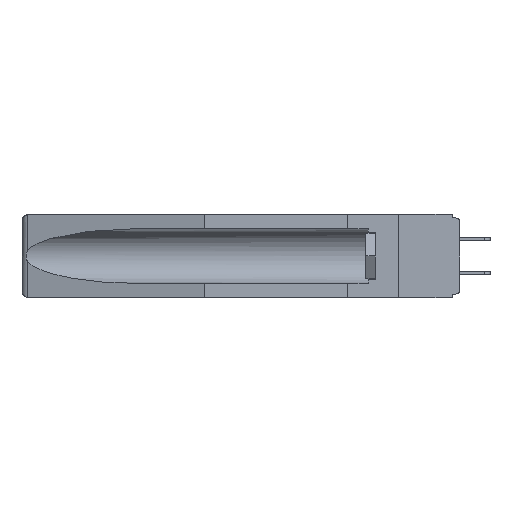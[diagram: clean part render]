
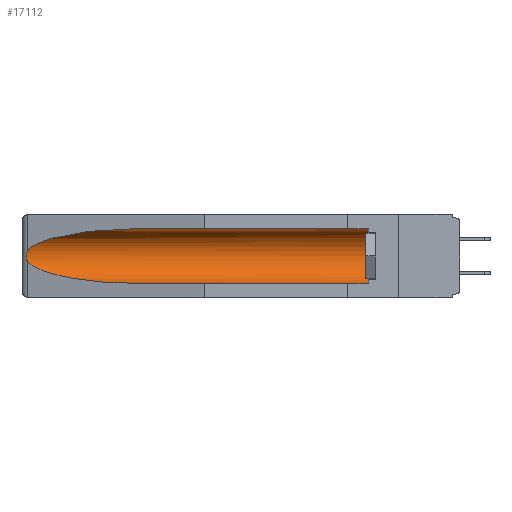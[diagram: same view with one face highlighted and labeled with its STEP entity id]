
A CAD part, left-side view. The second image highlights one B-rep face of the part: STEP entity #17112.
In plain terms, the highlighted cylindrical face has radius 2.857 mm (diameter 5.715 mm), a partial arc.
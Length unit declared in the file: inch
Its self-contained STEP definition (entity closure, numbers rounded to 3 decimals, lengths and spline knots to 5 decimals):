
#149 = VECTOR ( 'NONE', #13962, 39.37008 ) ;
#211 = CARTESIAN_POINT ( 'NONE',  ( 0.26537, 1.52718, -0.19328 ) ) ;
#336 = LINE ( 'NONE', #952, #14127 ) ;
#565 = EDGE_CURVE ( 'NONE', #11553, #15283, #336, .T. ) ;
#869 = CARTESIAN_POINT ( 'NONE',  ( 0.155, 1.07973, -0.284 ) ) ;
#952 = CARTESIAN_POINT ( 'NONE',  ( 0.155, -0.30754, -0.059 ) ) ;
#1368 = ORIENTED_EDGE ( 'NONE', *, *, #20794, .T. ) ;
#1974 = CARTESIAN_POINT ( 'NONE',  ( 0.26597, 1.5296, -0.19026 ) ) ;
#2362 = VERTEX_POINT ( 'NONE', #9225 ) ;
#2895 = AXIS2_PLACEMENT_3D ( 'NONE', #11987, #12065, #15499 ) ;
#2953 = DIRECTION ( 'NONE',  ( 0., 1., 0. ) ) ;
#3411 = ORIENTED_EDGE ( 'NONE', *, *, #19638, .T. ) ;
#3944 = DIRECTION ( 'NONE',  ( 0., 1., 0. ) ) ;
#4261 = ORIENTED_EDGE ( 'NONE', *, *, #10939, .F. ) ;
#4383 = CARTESIAN_POINT ( 'NONE',  ( 0.155, 1.07973, -0.059 ) ) ;
#4725 = CARTESIAN_POINT ( 'NONE',  ( 0.155, 0.126, -0.059 ) ) ;
#4789 = CARTESIAN_POINT ( 'NONE',  ( 0.25451, 1.48313, -0.24835 ) ) ;
#4915 = CARTESIAN_POINT ( 'NONE',  ( 0.26537, 1.52718, -0.14972 ) ) ;
#4972 = EDGE_CURVE ( 'NONE', #11870, #2362, #10192, .T. ) ;
#5327 = CARTESIAN_POINT ( 'NONE',  ( 0.2673, 1.5327, -0.16383 ) ) ;
#5405 = CARTESIAN_POINT ( 'NONE',  ( 0.2673, 1.53269, -0.17917 ) ) ;
#5622 = CARTESIAN_POINT ( 'NONE',  ( 0.26654, 1.53092, -0.15636 ) ) ;
#5827 = CARTESIAN_POINT ( 'NONE',  ( 0.155, -0.30754, -0.1715 ) ) ;
#6804 = CARTESIAN_POINT ( 'NONE',  ( 0.155, 1.07973, -0.284 ) ) ;
#7190 = CARTESIAN_POINT ( 'NONE',  ( 0.26537, 1.52718, -0.14972 ) ) ;
#7293 = ORIENTED_EDGE ( 'NONE', *, *, #565, .T. ) ;
#8412 = AXIS2_PLACEMENT_3D ( 'NONE', #5827, #3944, #18020 ) ;
#8425 = ORIENTED_EDGE ( 'NONE', *, *, #21726, .T. ) ;
#9023 = CARTESIAN_POINT ( 'NONE',  ( 0.2675, 1.53308, -0.17534 ) ) ;
#9225 = CARTESIAN_POINT ( 'NONE',  ( 0.26537, 1.52718, -0.19328 ) ) ;
#10192 = B_SPLINE_CURVE_WITH_KNOTS ( 'NONE', 3,
 ( #7190, #19563, #5622, #5327, #17592, #9023, #5405, #10769, #1974, #211 ),
 .UNSPECIFIED., .F., .F.,
 ( 4, 2, 2, 2, 4 ),
 ( 0., 0.00029, 0.00058, 0.00087, 0.00117 ),
 .UNSPECIFIED. ) ;
#10769 = CARTESIAN_POINT ( 'NONE',  ( 0.26655, 1.53094, -0.18657 ) ) ;
#10939 = EDGE_CURVE ( 'NONE', #21708, #21014, #15548, .T. ) ;
#11553 = VERTEX_POINT ( 'NONE', #4725 ) ;
#11870 = VERTEX_POINT ( 'NONE', #4915 ) ;
#11987 = CARTESIAN_POINT ( 'NONE',  ( 0.155, 0.126, -0.1715 ) ) ;
#12065 = DIRECTION ( 'NONE',  ( 0., -1., 0. ) ) ;
#13962 = DIRECTION ( 'NONE',  ( 0., 1., 0. ) ) ;
#14066 = FACE_OUTER_BOUND ( 'NONE', #15902, .T. ) ;
#14127 = VECTOR ( 'NONE', #2953, 39.37008 ) ;
#15283 = VERTEX_POINT ( 'NONE', #19220 ) ;
#15499 = DIRECTION ( 'NONE',  ( 0., 0., 1. ) ) ;
#15548 = LINE ( 'NONE', #22523, #149 ) ;
#15902 = EDGE_LOOP ( 'NONE', ( #3411, #18120, #8425, #4261, #1368, #7293 ) ) ;
#16937 =( BOUNDED_CURVE ( )  B_SPLINE_CURVE ( 3, ( #18769, #4789, #22269, #6804 ),
 .UNSPECIFIED., .F., .T. ) 
 B_SPLINE_CURVE_WITH_KNOTS ( ( 4, 4 ),
 ( 0.1948, 1.5708 ),
 .UNSPECIFIED. ) 
 CURVE ( )  GEOMETRIC_REPRESENTATION_ITEM ( )  RATIONAL_B_SPLINE_CURVE ( ( 1., 0.848, 0.848, 1. ) ) 
 REPRESENTATION_ITEM ( '' )  );
#17112 = ADVANCED_FACE ( 'NONE', ( #14066 ), #18167, .F. ) ;
#17592 = CARTESIAN_POINT ( 'NONE',  ( 0.2675, 1.53308, -0.16763 ) ) ;
#18020 = DIRECTION ( 'NONE',  ( 0., 0., 1. ) ) ;
#18120 = ORIENTED_EDGE ( 'NONE', *, *, #4972, .T. ) ;
#18167 = CYLINDRICAL_SURFACE ( 'NONE', #8412, 0.1125 ) ;
#18358 = CARTESIAN_POINT ( 'NONE',  ( 0.26537, 1.52718, -0.14972 ) ) ;
#18442 = CARTESIAN_POINT ( 'NONE',  ( 0.25451, 1.48313, -0.09465 ) ) ;
#18769 = CARTESIAN_POINT ( 'NONE',  ( 0.26537, 1.52718, -0.19328 ) ) ;
#18852 = CARTESIAN_POINT ( 'NONE',  ( 0.155, 0.126, -0.284 ) ) ;
#19220 = CARTESIAN_POINT ( 'NONE',  ( 0.155, 1.07973, -0.059 ) ) ;
#19563 = CARTESIAN_POINT ( 'NONE',  ( 0.26597, 1.52961, -0.15275 ) ) ;
#19638 = EDGE_CURVE ( 'NONE', #15283, #11870, #20781, .T. ) ;
#20781 =( BOUNDED_CURVE ( )  B_SPLINE_CURVE ( 3, ( #4383, #22094, #18442, #18358 ),
 .UNSPECIFIED., .F., .F. ) 
 B_SPLINE_CURVE_WITH_KNOTS ( ( 4, 4 ),
 ( 4.71239, 6.08839 ),
 .UNSPECIFIED. ) 
 CURVE ( )  GEOMETRIC_REPRESENTATION_ITEM ( )  RATIONAL_B_SPLINE_CURVE ( ( 1., 0.848, 0.848, 1. ) ) 
 REPRESENTATION_ITEM ( '' )  );
#20794 = EDGE_CURVE ( 'NONE', #21708, #11553, #21707, .T. ) ;
#21014 = VERTEX_POINT ( 'NONE', #869 ) ;
#21707 = CIRCLE ( 'NONE', #2895, 0.1125 ) ;
#21708 = VERTEX_POINT ( 'NONE', #18852 ) ;
#21726 = EDGE_CURVE ( 'NONE', #2362, #21014, #16937, .T. ) ;
#22094 = CARTESIAN_POINT ( 'NONE',  ( 0.21114, 1.30732, -0.059 ) ) ;
#22269 = CARTESIAN_POINT ( 'NONE',  ( 0.21114, 1.30732, -0.284 ) ) ;
#22523 = CARTESIAN_POINT ( 'NONE',  ( 0.155, -0.30754, -0.284 ) ) ;
